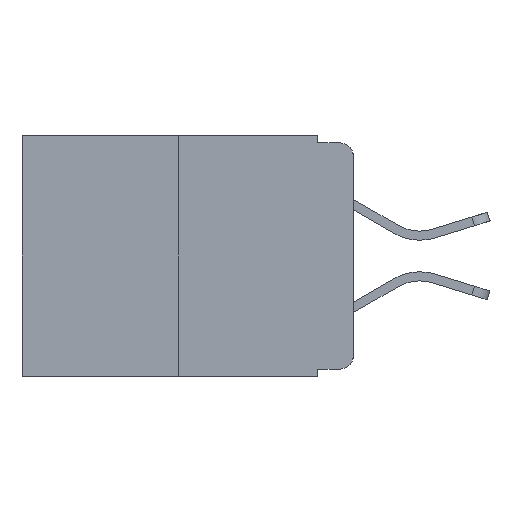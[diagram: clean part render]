
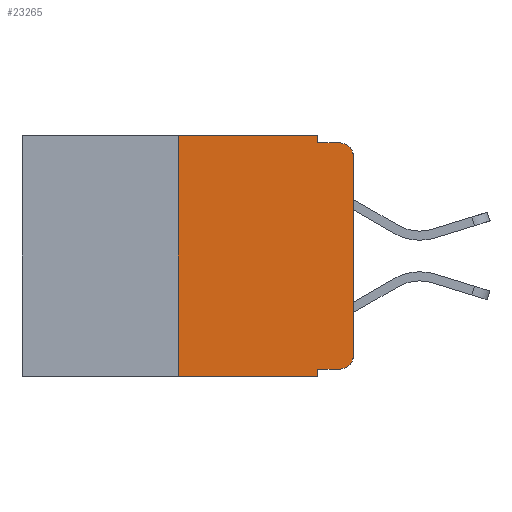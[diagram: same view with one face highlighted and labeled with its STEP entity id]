
A CAD part, left-side view. The second image highlights one B-rep face of the part: STEP entity #23265.
In plain terms, the highlighted planar face has unit normal (-1, 0, 0).
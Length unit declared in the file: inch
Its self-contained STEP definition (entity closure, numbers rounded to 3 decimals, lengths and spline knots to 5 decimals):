
#5 = VECTOR ( 'NONE', #4939, 39.37008 ) ;
#169 = VECTOR ( 'NONE', #5775, 39.37008 ) ;
#984 = VERTEX_POINT ( 'NONE', #4701 ) ;
#1488 = ORIENTED_EDGE ( 'NONE', *, *, #12429, .F. ) ;
#2821 = CARTESIAN_POINT ( 'NONE',  ( 0., 0.051, -0.01 ) ) ;
#2961 = ORIENTED_EDGE ( 'NONE', *, *, #9569, .T. ) ;
#3111 = VECTOR ( 'NONE', #8570, 39.37008 ) ;
#4128 = VECTOR ( 'NONE', #12511, 39.37008 ) ;
#4353 = EDGE_CURVE ( 'NONE', #984, #14428, #9005, .T. ) ;
#4406 = EDGE_LOOP ( 'NONE', ( #2961, #9609, #5305, #1488, #20889, #16695, #22580, #18383, #9906, #6184 ) ) ;
#4593 = VERTEX_POINT ( 'NONE', #13073 ) ;
#4701 = CARTESIAN_POINT ( 'NONE',  ( 0., 0.051, -0.333 ) ) ;
#4939 = DIRECTION ( 'NONE',  ( 0., 0., 1. ) ) ;
#4946 = CARTESIAN_POINT ( 'NONE',  ( 0., 0.02, -0.313 ) ) ;
#5305 = ORIENTED_EDGE ( 'NONE', *, *, #17312, .F. ) ;
#5324 = VECTOR ( 'NONE', #8656, 39.37008 ) ;
#5625 = LINE ( 'NONE', #19461, #5 ) ;
#5742 = LINE ( 'NONE', #21090, #10036 ) ;
#5775 = DIRECTION ( 'NONE',  ( 0., -1., 0. ) ) ;
#6184 = ORIENTED_EDGE ( 'NONE', *, *, #15041, .T. ) ;
#6328 = FACE_OUTER_BOUND ( 'NONE', #4406, .T. ) ;
#6588 = VERTEX_POINT ( 'NONE', #8240 ) ;
#6639 = CARTESIAN_POINT ( 'NONE',  ( 0., 0.473, 0. ) ) ;
#6723 = DIRECTION ( 'NONE',  ( 0., -1., 0. ) ) ;
#6812 = DIRECTION ( 'NONE',  ( 0., 0., -1. ) ) ;
#8053 = LINE ( 'NONE', #17601, #3111 ) ;
#8215 = VERTEX_POINT ( 'NONE', #8470 ) ;
#8240 = CARTESIAN_POINT ( 'NONE',  ( 0., 0.051, 0. ) ) ;
#8264 = VERTEX_POINT ( 'NONE', #15751 ) ;
#8470 = CARTESIAN_POINT ( 'NONE',  ( 0., 0., -0.313 ) ) ;
#8478 = PLANE ( 'NONE',  #12328 ) ;
#8493 = CARTESIAN_POINT ( 'NONE',  ( 0., 0.02, -0.333 ) ) ;
#8570 = DIRECTION ( 'NONE',  ( 0., 0., 1. ) ) ;
#8630 = DIRECTION ( 'NONE',  ( -1., 0., 0. ) ) ;
#8656 = DIRECTION ( 'NONE',  ( 0., -1., 0. ) ) ;
#9005 = LINE ( 'NONE', #23302, #4128 ) ;
#9209 = EDGE_CURVE ( 'NONE', #4593, #14428, #15464, .T. ) ;
#9333 = LINE ( 'NONE', #20511, #17808 ) ;
#9468 = CIRCLE ( 'NONE', #13567, 0.02 ) ;
#9569 = EDGE_CURVE ( 'NONE', #8215, #17170, #8053, .T. ) ;
#9609 = ORIENTED_EDGE ( 'NONE', *, *, #23300, .T. ) ;
#9714 = DIRECTION ( 'NONE',  ( 0., 0., -1. ) ) ;
#9906 = ORIENTED_EDGE ( 'NONE', *, *, #18777, .T. ) ;
#9985 = LINE ( 'NONE', #19811, #13673 ) ;
#10036 = VECTOR ( 'NONE', #6723, 39.37008 ) ;
#10185 = LINE ( 'NONE', #21287, #5324 ) ;
#10492 = CARTESIAN_POINT ( 'NONE',  ( 0., 0.051, -0.343 ) ) ;
#10591 = CARTESIAN_POINT ( 'NONE',  ( 0., 0.25, 0. ) ) ;
#10903 = CIRCLE ( 'NONE', #13612, 0.02 ) ;
#11291 = CARTESIAN_POINT ( 'NONE',  ( 0., 0.473, -0.343 ) ) ;
#12105 = DIRECTION ( 'NONE',  ( 0., 0., -1. ) ) ;
#12328 = AXIS2_PLACEMENT_3D ( 'NONE', #6639, #22909, #12105 ) ;
#12429 = EDGE_CURVE ( 'NONE', #6588, #15456, #9333, .T. ) ;
#12511 = DIRECTION ( 'NONE',  ( 0., 0., -1. ) ) ;
#13073 = CARTESIAN_POINT ( 'NONE',  ( 0., 0.25, -0.343 ) ) ;
#13567 = AXIS2_PLACEMENT_3D ( 'NONE', #19460, #8630, #21255 ) ;
#13612 = AXIS2_PLACEMENT_3D ( 'NONE', #4946, #17670, #6812 ) ;
#13673 = VECTOR ( 'NONE', #14478, 39.37008 ) ;
#14428 = VERTEX_POINT ( 'NONE', #10492 ) ;
#14478 = DIRECTION ( 'NONE',  ( 0., -1., 0. ) ) ;
#15041 = EDGE_CURVE ( 'NONE', #22754, #8215, #10903, .T. ) ;
#15456 = VERTEX_POINT ( 'NONE', #2821 ) ;
#15464 = LINE ( 'NONE', #11291, #169 ) ;
#15751 = CARTESIAN_POINT ( 'NONE',  ( 0., 0.02, -0.01 ) ) ;
#16695 = ORIENTED_EDGE ( 'NONE', *, *, #19393, .F. ) ;
#17170 = VERTEX_POINT ( 'NONE', #17694 ) ;
#17312 = EDGE_CURVE ( 'NONE', #15456, #8264, #9985, .T. ) ;
#17601 = CARTESIAN_POINT ( 'NONE',  ( 0., 0., 0. ) ) ;
#17670 = DIRECTION ( 'NONE',  ( -1., 0., 0. ) ) ;
#17694 = CARTESIAN_POINT ( 'NONE',  ( 0., 0., -0.03 ) ) ;
#17808 = VECTOR ( 'NONE', #9714, 39.37008 ) ;
#18383 = ORIENTED_EDGE ( 'NONE', *, *, #4353, .F. ) ;
#18466 = VERTEX_POINT ( 'NONE', #10591 ) ;
#18777 = EDGE_CURVE ( 'NONE', #984, #22754, #10185, .T. ) ;
#19393 = EDGE_CURVE ( 'NONE', #4593, #18466, #5625, .T. ) ;
#19460 = CARTESIAN_POINT ( 'NONE',  ( 0., 0.02, -0.03 ) ) ;
#19461 = CARTESIAN_POINT ( 'NONE',  ( 0., 0.25, 0. ) ) ;
#19811 = CARTESIAN_POINT ( 'NONE',  ( 0., 0.051, -0.01 ) ) ;
#20511 = CARTESIAN_POINT ( 'NONE',  ( 0., 0.051, 0. ) ) ;
#20889 = ORIENTED_EDGE ( 'NONE', *, *, #23274, .F. ) ;
#21090 = CARTESIAN_POINT ( 'NONE',  ( 0., 0.473, 0. ) ) ;
#21255 = DIRECTION ( 'NONE',  ( 0., 0., -1. ) ) ;
#21287 = CARTESIAN_POINT ( 'NONE',  ( 0., 0.051, -0.333 ) ) ;
#22580 = ORIENTED_EDGE ( 'NONE', *, *, #9209, .T. ) ;
#22754 = VERTEX_POINT ( 'NONE', #8493 ) ;
#22909 = DIRECTION ( 'NONE',  ( 1., 0., 0. ) ) ;
#23265 = ADVANCED_FACE ( 'NONE', ( #6328 ), #8478, .F. ) ;
#23274 = EDGE_CURVE ( 'NONE', #18466, #6588, #5742, .T. ) ;
#23300 = EDGE_CURVE ( 'NONE', #17170, #8264, #9468, .T. ) ;
#23302 = CARTESIAN_POINT ( 'NONE',  ( 0., 0.051, 0. ) ) ;
